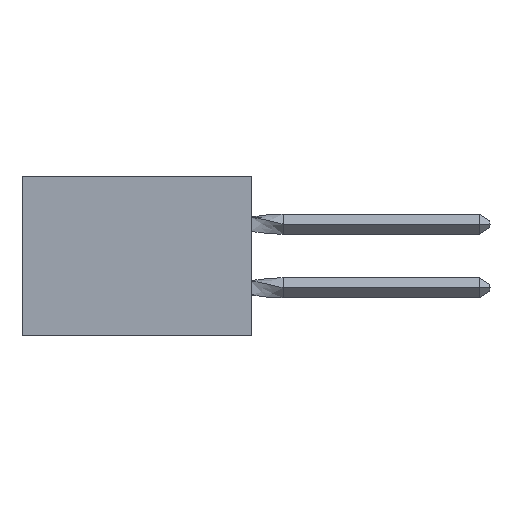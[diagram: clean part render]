
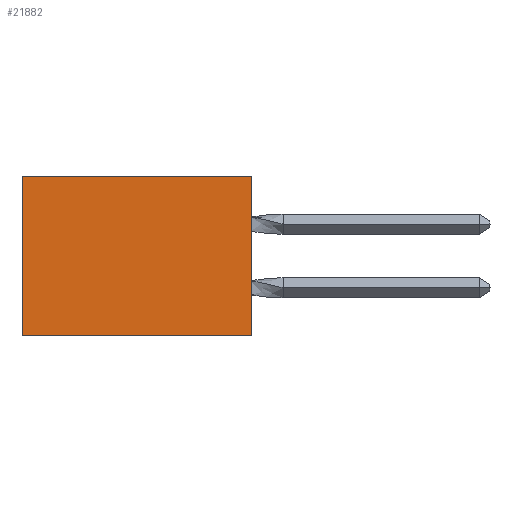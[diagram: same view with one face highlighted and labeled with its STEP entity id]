
A CAD part, left-side view. The second image highlights one B-rep face of the part: STEP entity #21882.
In plain terms, the highlighted planar face has unit normal (-1, 0, 0).
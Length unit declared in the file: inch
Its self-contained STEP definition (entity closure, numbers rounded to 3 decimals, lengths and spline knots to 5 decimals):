
#1676 = EDGE_CURVE ( 'NONE', #11887, #8088, #14210, .T. ) ;
#1857 = VECTOR ( 'NONE', #17520, 39.37008 ) ;
#1934 = LINE ( 'NONE', #14158, #11542 ) ;
#2521 = EDGE_CURVE ( 'NONE', #21008, #11887, #4390, .T. ) ;
#3698 = CARTESIAN_POINT ( 'NONE',  ( 0.305, 0., -0.5 ) ) ;
#4390 = LINE ( 'NONE', #18341, #6848 ) ;
#4917 = LINE ( 'NONE', #9440, #16466 ) ;
#5645 = CARTESIAN_POINT ( 'NONE',  ( 0.305, 0.72, 0. ) ) ;
#5841 = ORIENTED_EDGE ( 'NONE', *, *, #2521, .F. ) ;
#5855 = EDGE_CURVE ( 'NONE', #21008, #12802, #1934, .T. ) ;
#6848 = VECTOR ( 'NONE', #15083, 39.37008 ) ;
#8088 = VERTEX_POINT ( 'NONE', #19362 ) ;
#9388 = ORIENTED_EDGE ( 'NONE', *, *, #5855, .T. ) ;
#9440 = CARTESIAN_POINT ( 'NONE',  ( 0.305, 0.72, -0.5 ) ) ;
#9761 = EDGE_LOOP ( 'NONE', ( #21938, #11599, #5841, #9388 ) ) ;
#10740 = PLANE ( 'NONE',  #21836 ) ;
#10894 = EDGE_CURVE ( 'NONE', #12802, #8088, #4917, .T. ) ;
#11215 = DIRECTION ( 'NONE',  ( 0., 0., -1. ) ) ;
#11542 = VECTOR ( 'NONE', #17471, 39.37008 ) ;
#11599 = ORIENTED_EDGE ( 'NONE', *, *, #1676, .F. ) ;
#11846 = CARTESIAN_POINT ( 'NONE',  ( 0.305, 0., 0. ) ) ;
#11887 = VERTEX_POINT ( 'NONE', #19720 ) ;
#12440 = DIRECTION ( 'NONE',  ( 0., 0., -1. ) ) ;
#12788 = FACE_OUTER_BOUND ( 'NONE', #9761, .T. ) ;
#12802 = VERTEX_POINT ( 'NONE', #5645 ) ;
#14158 = CARTESIAN_POINT ( 'NONE',  ( 0.305, 0., 0. ) ) ;
#14210 = LINE ( 'NONE', #3698, #1857 ) ;
#15083 = DIRECTION ( 'NONE',  ( 0., 0., -1. ) ) ;
#15947 = CARTESIAN_POINT ( 'NONE',  ( 0.305, 0., -0.5 ) ) ;
#16466 = VECTOR ( 'NONE', #11215, 39.37008 ) ;
#17471 = DIRECTION ( 'NONE',  ( 0., 1., 0. ) ) ;
#17520 = DIRECTION ( 'NONE',  ( 0., 1., 0. ) ) ;
#18341 = CARTESIAN_POINT ( 'NONE',  ( 0.305, 0., -0.5 ) ) ;
#19362 = CARTESIAN_POINT ( 'NONE',  ( 0.305, 0.72, -0.5 ) ) ;
#19720 = CARTESIAN_POINT ( 'NONE',  ( 0.305, 0., -0.5 ) ) ;
#21008 = VERTEX_POINT ( 'NONE', #11846 ) ;
#21202 = DIRECTION ( 'NONE',  ( 1., 0., 0. ) ) ;
#21836 = AXIS2_PLACEMENT_3D ( 'NONE', #15947, #21202, #12440 ) ;
#21882 = ADVANCED_FACE ( 'NONE', ( #12788 ), #10740, .F. ) ;
#21938 = ORIENTED_EDGE ( 'NONE', *, *, #10894, .T. ) ;
